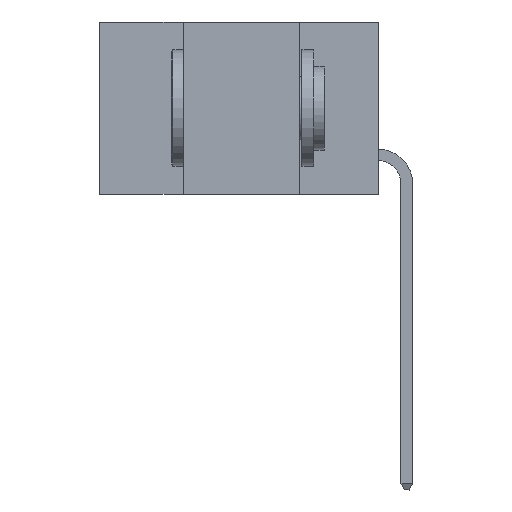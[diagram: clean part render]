
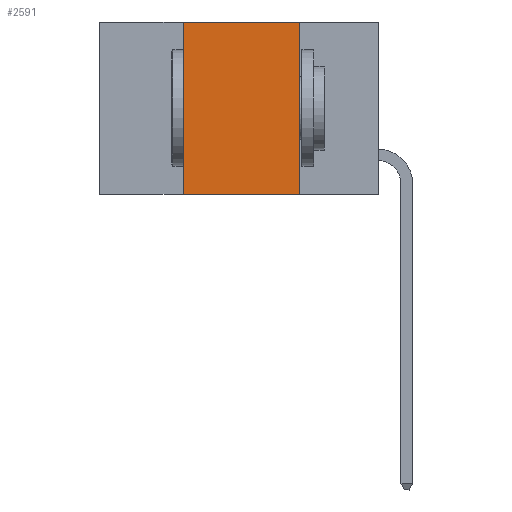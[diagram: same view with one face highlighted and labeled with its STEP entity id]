
A CAD part, left-side view. The second image highlights one B-rep face of the part: STEP entity #2591.
In plain terms, the highlighted planar face has unit normal (-1, 0, 0).
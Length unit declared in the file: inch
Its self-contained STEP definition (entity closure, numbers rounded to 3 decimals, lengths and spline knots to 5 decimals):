
#925 = EDGE_CURVE ( 'NONE', #20305, #10616, #2979, .T. ) ;
#2591 = ADVANCED_FACE ( 'NONE', ( #18347 ), #15424, .F. ) ;
#2887 = ORIENTED_EDGE ( 'NONE', *, *, #925, .T. ) ;
#2979 = LINE ( 'NONE', #18330, #6409 ) ;
#3956 = CARTESIAN_POINT ( 'NONE',  ( 0., 0.42, 0. ) ) ;
#4101 = VECTOR ( 'NONE', #14033, 39.37008 ) ;
#4571 = CARTESIAN_POINT ( 'NONE',  ( 0., 0.42, -0.37 ) ) ;
#4801 = DIRECTION ( 'NONE',  ( 0., 0., -1. ) ) ;
#4851 = DIRECTION ( 'NONE',  ( 1., 0., 0. ) ) ;
#4874 = CARTESIAN_POINT ( 'NONE',  ( 0., 0.6, 0. ) ) ;
#4917 = DIRECTION ( 'NONE',  ( 0., 0., 1. ) ) ;
#5472 = CARTESIAN_POINT ( 'NONE',  ( 0., 0.17, -0.37 ) ) ;
#5552 = EDGE_CURVE ( 'NONE', #20305, #11280, #9706, .T. ) ;
#5579 = EDGE_CURVE ( 'NONE', #11280, #6927, #8646, .T. ) ;
#6409 = VECTOR ( 'NONE', #19926, 39.37008 ) ;
#6927 = VERTEX_POINT ( 'NONE', #11354 ) ;
#8283 = ORIENTED_EDGE ( 'NONE', *, *, #9694, .F. ) ;
#8646 = LINE ( 'NONE', #16339, #4101 ) ;
#9505 = EDGE_LOOP ( 'NONE', ( #8283, #12987, #11147, #2887 ) ) ;
#9694 = EDGE_CURVE ( 'NONE', #6927, #10616, #17571, .T. ) ;
#9706 = LINE ( 'NONE', #15464, #17451 ) ;
#10616 = VERTEX_POINT ( 'NONE', #5472 ) ;
#11147 = ORIENTED_EDGE ( 'NONE', *, *, #5552, .F. ) ;
#11280 = VERTEX_POINT ( 'NONE', #3956 ) ;
#11354 = CARTESIAN_POINT ( 'NONE',  ( 0., 0.17, 0. ) ) ;
#12987 = ORIENTED_EDGE ( 'NONE', *, *, #5579, .F. ) ;
#13202 = VECTOR ( 'NONE', #16334, 39.37008 ) ;
#14033 = DIRECTION ( 'NONE',  ( 0., -1., 0. ) ) ;
#15424 = PLANE ( 'NONE',  #19259 ) ;
#15464 = CARTESIAN_POINT ( 'NONE',  ( 0., 0.42, 0. ) ) ;
#16334 = DIRECTION ( 'NONE',  ( 0., 0., -1. ) ) ;
#16339 = CARTESIAN_POINT ( 'NONE',  ( 0., 0.6, 0. ) ) ;
#17451 = VECTOR ( 'NONE', #4917, 39.37008 ) ;
#17571 = LINE ( 'NONE', #17880, #13202 ) ;
#17880 = CARTESIAN_POINT ( 'NONE',  ( 0., 0.17, 0. ) ) ;
#18330 = CARTESIAN_POINT ( 'NONE',  ( 0., 0.6, -0.37 ) ) ;
#18347 = FACE_OUTER_BOUND ( 'NONE', #9505, .T. ) ;
#19259 = AXIS2_PLACEMENT_3D ( 'NONE', #4874, #4851, #4801 ) ;
#19926 = DIRECTION ( 'NONE',  ( 0., -1., 0. ) ) ;
#20305 = VERTEX_POINT ( 'NONE', #4571 ) ;
